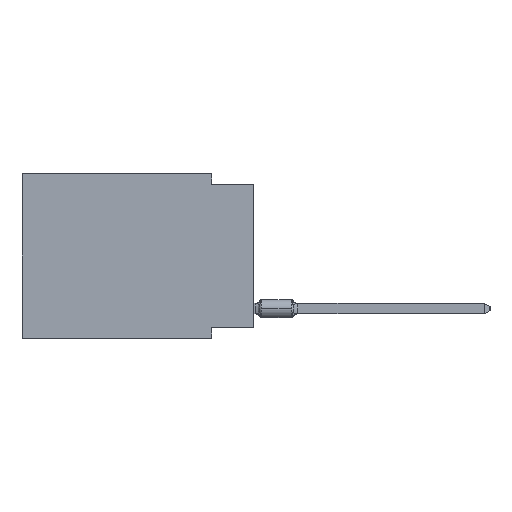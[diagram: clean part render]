
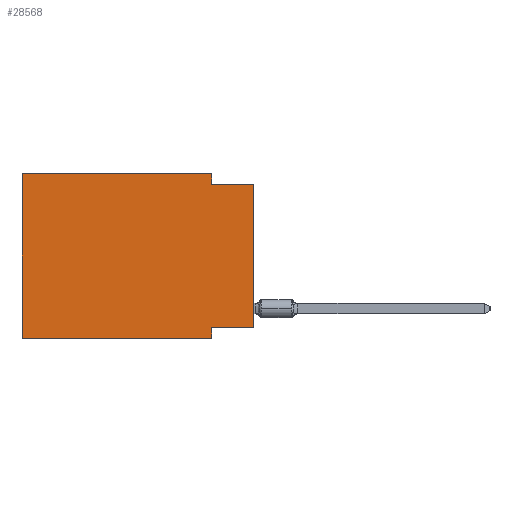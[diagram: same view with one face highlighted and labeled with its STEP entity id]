
A CAD part, left-side view. The second image highlights one B-rep face of the part: STEP entity #28568.
In plain terms, the highlighted planar face has unit normal (-1, 0, 0).
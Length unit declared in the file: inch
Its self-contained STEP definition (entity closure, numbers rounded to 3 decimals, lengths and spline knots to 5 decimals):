
#887 = VERTEX_POINT ( 'NONE', #9588 ) ;
#1439 = DIRECTION ( 'NONE',  ( 0., 0., -1. ) ) ;
#1642 = DIRECTION ( 'NONE',  ( 0., 0., 1. ) ) ;
#1860 = EDGE_CURVE ( 'NONE', #12086, #22165, #10864, .T. ) ;
#2624 = AXIS2_PLACEMENT_3D ( 'NONE', #20487, #10894, #1439 ) ;
#3154 = VECTOR ( 'NONE', #15470, 39.37008 ) ;
#3234 = CARTESIAN_POINT ( 'NONE',  ( 0., 0.55, -0.39 ) ) ;
#3402 = VERTEX_POINT ( 'NONE', #16093 ) ;
#4020 = CARTESIAN_POINT ( 'NONE',  ( 0., 0.1, -0.365 ) ) ;
#5306 = VECTOR ( 'NONE', #14683, 39.37008 ) ;
#5546 = EDGE_CURVE ( 'NONE', #16751, #18072, #22136, .T. ) ;
#6210 = DIRECTION ( 'NONE',  ( 0., 1., 0. ) ) ;
#6443 = LINE ( 'NONE', #18226, #24518 ) ;
#6651 = DIRECTION ( 'NONE',  ( 0., -1., 0. ) ) ;
#6986 = VECTOR ( 'NONE', #6651, 39.37008 ) ;
#7393 = CARTESIAN_POINT ( 'NONE',  ( 0., 0.1, -0.39 ) ) ;
#7531 = VERTEX_POINT ( 'NONE', #15393 ) ;
#9588 = CARTESIAN_POINT ( 'NONE',  ( 0., 0.1, 0. ) ) ;
#9880 = LINE ( 'NONE', #7393, #5306 ) ;
#9923 = EDGE_CURVE ( 'NONE', #887, #7531, #6443, .T. ) ;
#9928 = EDGE_CURVE ( 'NONE', #16751, #23197, #13571, .T. ) ;
#10172 = CARTESIAN_POINT ( 'NONE',  ( 0., 0.55, -0.39 ) ) ;
#10864 = LINE ( 'NONE', #27719, #12163 ) ;
#10894 = DIRECTION ( 'NONE',  ( 1., 0., 0. ) ) ;
#12086 = VERTEX_POINT ( 'NONE', #21720 ) ;
#12163 = VECTOR ( 'NONE', #6210, 39.37008 ) ;
#12251 = ORIENTED_EDGE ( 'NONE', *, *, #23048, .F. ) ;
#13571 = LINE ( 'NONE', #24867, #25506 ) ;
#13835 = DIRECTION ( 'NONE',  ( 0., -1., 0. ) ) ;
#14045 = EDGE_CURVE ( 'NONE', #22165, #18072, #9880, .T. ) ;
#14683 = DIRECTION ( 'NONE',  ( 0., 0., -1. ) ) ;
#14709 = EDGE_CURVE ( 'NONE', #12086, #3402, #28042, .T. ) ;
#15393 = CARTESIAN_POINT ( 'NONE',  ( 0., 0.1, -0.025 ) ) ;
#15470 = DIRECTION ( 'NONE',  ( 0., -1., 0. ) ) ;
#16093 = CARTESIAN_POINT ( 'NONE',  ( 0., 0., -0.025 ) ) ;
#16751 = VERTEX_POINT ( 'NONE', #10172 ) ;
#17369 = ORIENTED_EDGE ( 'NONE', *, *, #14045, .F. ) ;
#17715 = VECTOR ( 'NONE', #28186, 39.37008 ) ;
#18014 = FACE_OUTER_BOUND ( 'NONE', #20771, .T. ) ;
#18072 = VERTEX_POINT ( 'NONE', #24443 ) ;
#18119 = ORIENTED_EDGE ( 'NONE', *, *, #14709, .T. ) ;
#18226 = CARTESIAN_POINT ( 'NONE',  ( 0., 0.1, 0. ) ) ;
#18694 = EDGE_CURVE ( 'NONE', #23197, #887, #23727, .T. ) ;
#18761 = CARTESIAN_POINT ( 'NONE',  ( 0., 0., 0. ) ) ;
#18878 = CARTESIAN_POINT ( 'NONE',  ( 0., 0.55, 0. ) ) ;
#19751 = ORIENTED_EDGE ( 'NONE', *, *, #18694, .F. ) ;
#20400 = ORIENTED_EDGE ( 'NONE', *, *, #9923, .F. ) ;
#20487 = CARTESIAN_POINT ( 'NONE',  ( 0., 0.55, 0. ) ) ;
#20600 = CARTESIAN_POINT ( 'NONE',  ( 0., 0., -0.025 ) ) ;
#20771 = EDGE_LOOP ( 'NONE', ( #18119, #12251, #20400, #19751, #25309, #27498, #17369, #23631 ) ) ;
#21720 = CARTESIAN_POINT ( 'NONE',  ( 0., 0., -0.365 ) ) ;
#22136 = LINE ( 'NONE', #3234, #3154 ) ;
#22165 = VERTEX_POINT ( 'NONE', #4020 ) ;
#23048 = EDGE_CURVE ( 'NONE', #7531, #3402, #27861, .T. ) ;
#23116 = PLANE ( 'NONE',  #2624 ) ;
#23197 = VERTEX_POINT ( 'NONE', #18878 ) ;
#23424 = CARTESIAN_POINT ( 'NONE',  ( 0., 0.55, 0. ) ) ;
#23631 = ORIENTED_EDGE ( 'NONE', *, *, #1860, .F. ) ;
#23727 = LINE ( 'NONE', #23424, #27636 ) ;
#24443 = CARTESIAN_POINT ( 'NONE',  ( 0., 0.1, -0.39 ) ) ;
#24518 = VECTOR ( 'NONE', #27813, 39.37008 ) ;
#24867 = CARTESIAN_POINT ( 'NONE',  ( 0., 0.55, 0. ) ) ;
#25309 = ORIENTED_EDGE ( 'NONE', *, *, #9928, .F. ) ;
#25506 = VECTOR ( 'NONE', #1642, 39.37008 ) ;
#27498 = ORIENTED_EDGE ( 'NONE', *, *, #5546, .T. ) ;
#27636 = VECTOR ( 'NONE', #13835, 39.37008 ) ;
#27719 = CARTESIAN_POINT ( 'NONE',  ( 0., 0., -0.365 ) ) ;
#27813 = DIRECTION ( 'NONE',  ( 0., 0., -1. ) ) ;
#27861 = LINE ( 'NONE', #20600, #6986 ) ;
#28042 = LINE ( 'NONE', #18761, #17715 ) ;
#28186 = DIRECTION ( 'NONE',  ( 0., 0., 1. ) ) ;
#28568 = ADVANCED_FACE ( 'NONE', ( #18014 ), #23116, .F. ) ;
